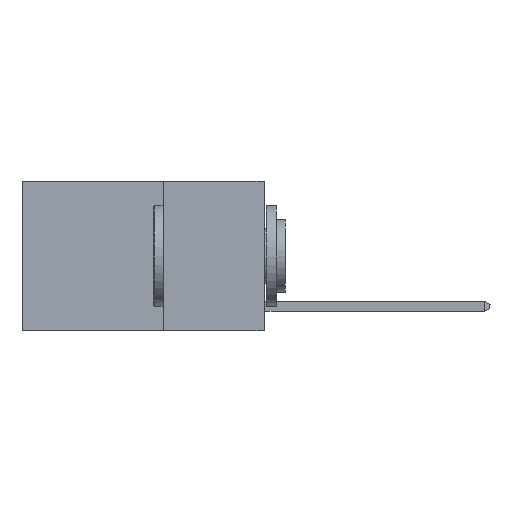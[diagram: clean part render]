
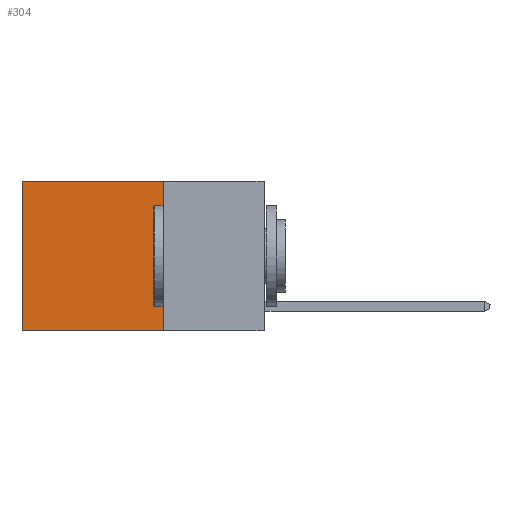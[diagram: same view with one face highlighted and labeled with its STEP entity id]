
A CAD part, left-side view. The second image highlights one B-rep face of the part: STEP entity #304.
In plain terms, the highlighted planar face has unit normal (-1, 0, 0).
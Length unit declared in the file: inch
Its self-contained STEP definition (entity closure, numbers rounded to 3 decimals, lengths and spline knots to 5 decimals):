
#10 = VECTOR ( 'NONE', #19337, 39.37008 ) ;
#116 = EDGE_CURVE ( 'NONE', #11397, #3649, #8557, .T. ) ;
#304 = ADVANCED_FACE ( 'NONE', ( #17442 ), #11314, .F. ) ;
#2759 = DIRECTION ( 'NONE',  ( 0., 0., -1. ) ) ;
#2862 = CARTESIAN_POINT ( 'NONE',  ( 0.2625, 0.25, 0. ) ) ;
#3649 = VERTEX_POINT ( 'NONE', #25718 ) ;
#4288 = DIRECTION ( 'NONE',  ( 0., 0., -1. ) ) ;
#4823 = LINE ( 'NONE', #7546, #15770 ) ;
#4871 = CARTESIAN_POINT ( 'NONE',  ( 0.2625, 0.25, 0. ) ) ;
#5219 = CARTESIAN_POINT ( 'NONE',  ( 0.2625, 0.25, 0. ) ) ;
#6558 = DIRECTION ( 'NONE',  ( 1., 0., 0. ) ) ;
#7444 = VERTEX_POINT ( 'NONE', #2862 ) ;
#7480 = EDGE_CURVE ( 'NONE', #19873, #3649, #4823, .T. ) ;
#7546 = CARTESIAN_POINT ( 'NONE',  ( 0.2625, 0.25, -0.37 ) ) ;
#7725 = AXIS2_PLACEMENT_3D ( 'NONE', #4871, #6558, #4288 ) ;
#8557 = LINE ( 'NONE', #9645, #17807 ) ;
#9645 = CARTESIAN_POINT ( 'NONE',  ( 0.2625, 0.6, 0. ) ) ;
#10472 = CARTESIAN_POINT ( 'NONE',  ( 0.2625, 0.25, 0. ) ) ;
#11197 = ORIENTED_EDGE ( 'NONE', *, *, #116, .T. ) ;
#11314 = PLANE ( 'NONE',  #7725 ) ;
#11397 = VERTEX_POINT ( 'NONE', #20912 ) ;
#11666 = DIRECTION ( 'NONE',  ( 0., 1., 0. ) ) ;
#13563 = ORIENTED_EDGE ( 'NONE', *, *, #18464, .F. ) ;
#14463 = ORIENTED_EDGE ( 'NONE', *, *, #7480, .F. ) ;
#15770 = VECTOR ( 'NONE', #11666, 39.37008 ) ;
#17442 = FACE_OUTER_BOUND ( 'NONE', #25799, .T. ) ;
#17617 = EDGE_CURVE ( 'NONE', #7444, #11397, #19497, .T. ) ;
#17807 = VECTOR ( 'NONE', #2759, 39.37008 ) ;
#18464 = EDGE_CURVE ( 'NONE', #7444, #19873, #26919, .T. ) ;
#19337 = DIRECTION ( 'NONE',  ( 0., 0., -1. ) ) ;
#19497 = LINE ( 'NONE', #5219, #19843 ) ;
#19843 = VECTOR ( 'NONE', #26662, 39.37008 ) ;
#19873 = VERTEX_POINT ( 'NONE', #25476 ) ;
#20912 = CARTESIAN_POINT ( 'NONE',  ( 0.2625, 0.6, 0. ) ) ;
#25476 = CARTESIAN_POINT ( 'NONE',  ( 0.2625, 0.25, -0.37 ) ) ;
#25655 = ORIENTED_EDGE ( 'NONE', *, *, #17617, .T. ) ;
#25718 = CARTESIAN_POINT ( 'NONE',  ( 0.2625, 0.6, -0.37 ) ) ;
#25799 = EDGE_LOOP ( 'NONE', ( #11197, #14463, #13563, #25655 ) ) ;
#26662 = DIRECTION ( 'NONE',  ( 0., 1., 0. ) ) ;
#26919 = LINE ( 'NONE', #10472, #10 ) ;
